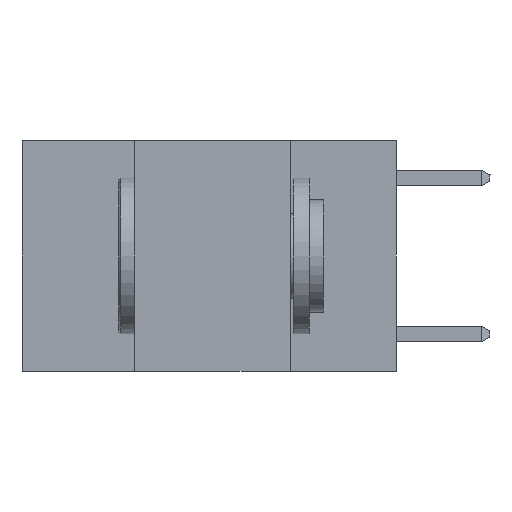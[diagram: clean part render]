
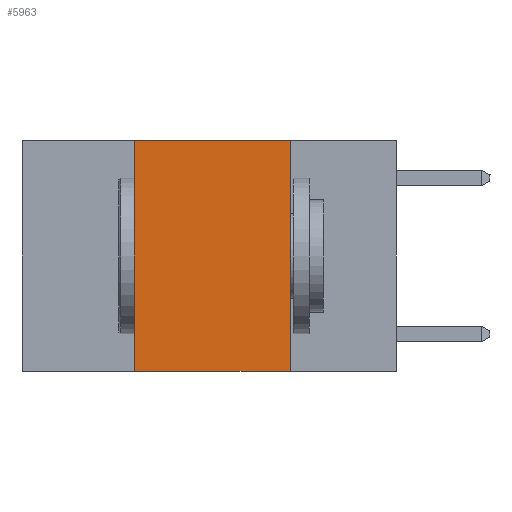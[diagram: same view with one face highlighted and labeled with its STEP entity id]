
A CAD part, left-side view. The second image highlights one B-rep face of the part: STEP entity #5963.
In plain terms, the highlighted planar face has unit normal (-1, 0, 0).
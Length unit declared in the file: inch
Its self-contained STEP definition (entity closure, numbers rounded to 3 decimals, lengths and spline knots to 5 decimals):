
#237 = CARTESIAN_POINT ( 'NONE',  ( 0., 0.42, 0. ) ) ;
#1041 = DIRECTION ( 'NONE',  ( 0., -1., 0. ) ) ;
#1811 = LINE ( 'NONE', #237, #6539 ) ;
#2358 = CARTESIAN_POINT ( 'NONE',  ( 0., 0.17, -0.37 ) ) ;
#3155 = CARTESIAN_POINT ( 'NONE',  ( 0., 0.6, -0.37 ) ) ;
#3431 = VERTEX_POINT ( 'NONE', #4707 ) ;
#3566 = AXIS2_PLACEMENT_3D ( 'NONE', #7327, #5560, #3741 ) ;
#3741 = DIRECTION ( 'NONE',  ( 0., 0., -1. ) ) ;
#3743 = EDGE_CURVE ( 'NONE', #6663, #4793, #7863, .T. ) ;
#3836 = ORIENTED_EDGE ( 'NONE', *, *, #8215, .F. ) ;
#4447 = CARTESIAN_POINT ( 'NONE',  ( 0., 0.6, 0. ) ) ;
#4707 = CARTESIAN_POINT ( 'NONE',  ( 0., 0.42, -0.37 ) ) ;
#4788 = DIRECTION ( 'NONE',  ( 0., -1., 0. ) ) ;
#4793 = VERTEX_POINT ( 'NONE', #5559 ) ;
#5387 = FACE_OUTER_BOUND ( 'NONE', #10366, .T. ) ;
#5559 = CARTESIAN_POINT ( 'NONE',  ( 0., 0.17, 0. ) ) ;
#5560 = DIRECTION ( 'NONE',  ( 1., 0., 0. ) ) ;
#5661 = VERTEX_POINT ( 'NONE', #2358 ) ;
#5963 = ADVANCED_FACE ( 'NONE', ( #5387 ), #8056, .F. ) ;
#6157 = DIRECTION ( 'NONE',  ( 0., 0., 1. ) ) ;
#6539 = VECTOR ( 'NONE', #6157, 39.37008 ) ;
#6663 = VERTEX_POINT ( 'NONE', #8916 ) ;
#7294 = LINE ( 'NONE', #3155, #8689 ) ;
#7327 = CARTESIAN_POINT ( 'NONE',  ( 0., 0.6, 0. ) ) ;
#7354 = VECTOR ( 'NONE', #8365, 39.37008 ) ;
#7420 = LINE ( 'NONE', #8987, #7354 ) ;
#7863 = LINE ( 'NONE', #4447, #10082 ) ;
#7911 = EDGE_CURVE ( 'NONE', #3431, #5661, #7294, .T. ) ;
#8056 = PLANE ( 'NONE',  #3566 ) ;
#8215 = EDGE_CURVE ( 'NONE', #3431, #6663, #1811, .T. ) ;
#8345 = ORIENTED_EDGE ( 'NONE', *, *, #3743, .F. ) ;
#8365 = DIRECTION ( 'NONE',  ( 0., 0., -1. ) ) ;
#8578 = ORIENTED_EDGE ( 'NONE', *, *, #7911, .T. ) ;
#8689 = VECTOR ( 'NONE', #4788, 39.37008 ) ;
#8916 = CARTESIAN_POINT ( 'NONE',  ( 0., 0.42, 0. ) ) ;
#8987 = CARTESIAN_POINT ( 'NONE',  ( 0., 0.17, 0. ) ) ;
#10082 = VECTOR ( 'NONE', #1041, 39.37008 ) ;
#10366 = EDGE_LOOP ( 'NONE', ( #10964, #8345, #3836, #8578 ) ) ;
#10589 = EDGE_CURVE ( 'NONE', #4793, #5661, #7420, .T. ) ;
#10964 = ORIENTED_EDGE ( 'NONE', *, *, #10589, .F. ) ;
